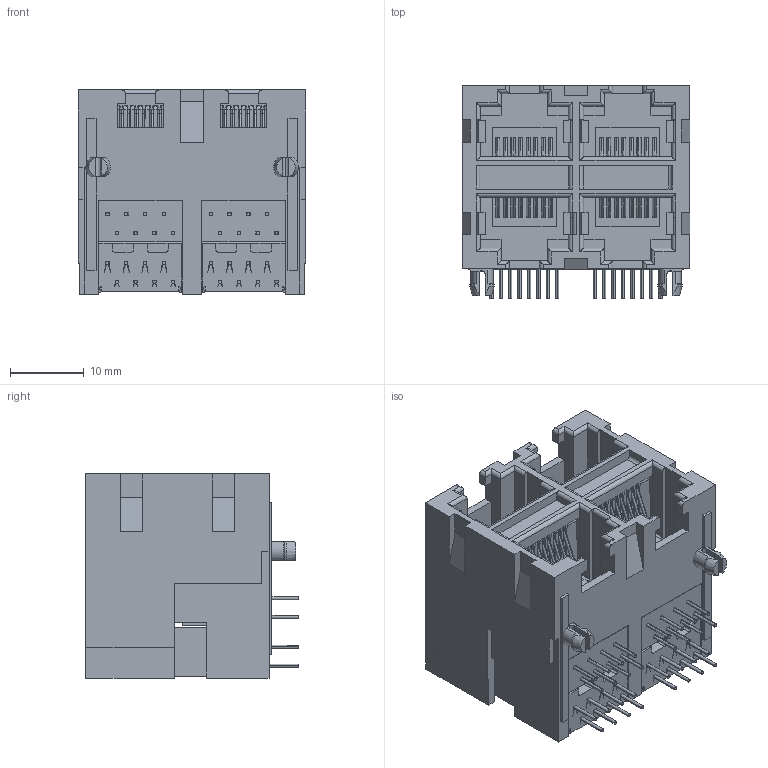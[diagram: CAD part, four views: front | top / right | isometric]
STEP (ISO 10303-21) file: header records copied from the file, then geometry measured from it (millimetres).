
FILE_DESCRIPTION (( 'STEP AP203' ), '1' );
FILE_NAME ('RJ9F048832P00021.STEP', '2020-01-15T15:43:54', ( '' ), ( '' ), 'SwSTEP 2.0', 'SolidWorks 2016', '' );
FILE_SCHEMA (( 'CONFIG_CONTROL_DESIGN' ));
Length unit declared in the file: millimetre
Products named in the file (6): RJ9F048832P00021; 9F Contacts Lower; 9F Contacts Upper; 9F Contact Lock Upper; 9F Contact Lock Lower; 9F Insulator
Assembly tree (9 placements, depth 2):
  RJ9F048832P00021
    9F Insulator
    9F Contact Lock Lower  x2
    9F Contact Lock Upper  x2
    9F Contacts Lower  x2
    9F Contacts Upper  x2
Bounding box: 30.74 x 28.71 x 27.6 mm (x, y, z)
Volume: 11763.1 mm3; surface area: 19773.9 mm2
Topology: 37 solids, 37 shells, 2810 faces, 7493 edges, 4689 vertices
Faces by surface type: plane 1899, cylinder 557, torus 268, cone 74, bspline 12
Entity records: 56857 total; most frequent: CARTESIAN_POINT 14058, ORIENTED_EDGE 9370, DIRECTION 7882, EDGE_CURVE 4685, LINE 3114, VECTOR 3114, VERTEX_POINT 2957, AXIS2_PLACEMENT_3D 2384
